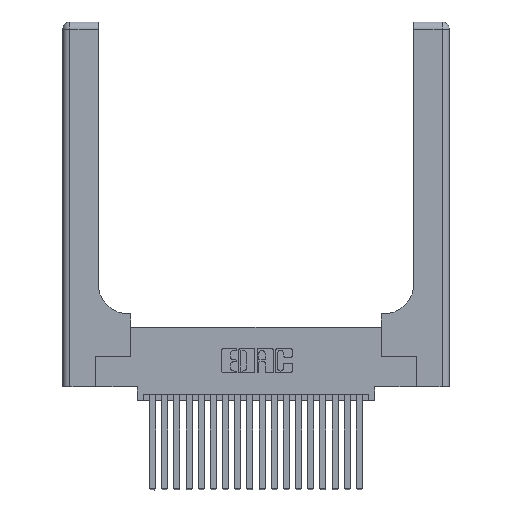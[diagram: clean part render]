
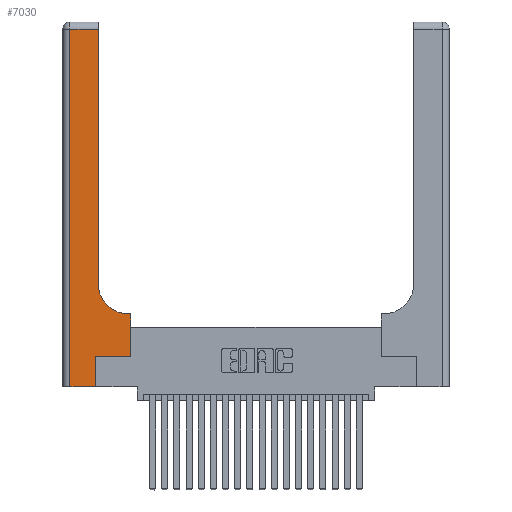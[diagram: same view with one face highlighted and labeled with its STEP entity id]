
A CAD part, top view. The second image highlights one B-rep face of the part: STEP entity #7030.
In plain terms, the highlighted planar face has unit normal (0, 0, 1).
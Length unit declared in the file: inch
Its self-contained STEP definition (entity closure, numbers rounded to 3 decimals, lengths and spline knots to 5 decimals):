
#413 = EDGE_CURVE ( 'NONE', #3244, #18240, #7618, .T. ) ;
#979 = DIRECTION ( 'NONE',  ( 0., 0., -1. ) ) ;
#2096 = CARTESIAN_POINT ( 'NONE',  ( 0.2915, 0.6, 0.37 ) ) ;
#2308 = DIRECTION ( 'NONE',  ( 0., 0., -1. ) ) ;
#2321 = DIRECTION ( 'NONE',  ( 0., 1., 0. ) ) ;
#3053 = EDGE_CURVE ( 'NONE', #18240, #21819, #3371, .T. ) ;
#3215 = EDGE_CURVE ( 'NONE', #21819, #20102, #10783, .T. ) ;
#3244 = VERTEX_POINT ( 'NONE', #16145 ) ;
#3371 = LINE ( 'NONE', #14045, #15663 ) ;
#3552 = VERTEX_POINT ( 'NONE', #8536 ) ;
#3729 = CARTESIAN_POINT ( 'NONE',  ( 0.269, 0., 0.37 ) ) ;
#3808 = DIRECTION ( 'NONE',  ( 0., 1., 0. ) ) ;
#4030 = LINE ( 'NONE', #7240, #22029 ) ;
#4136 = DIRECTION ( 'NONE',  ( -1., 0., 0. ) ) ;
#4292 = CARTESIAN_POINT ( 'NONE',  ( 0.2915, 0.85, 0.37 ) ) ;
#4666 = VERTEX_POINT ( 'NONE', #6856 ) ;
#5130 = CIRCLE ( 'NONE', #10018, 0.25 ) ;
#5564 = LINE ( 'NONE', #19434, #20297 ) ;
#5689 = CARTESIAN_POINT ( 'NONE',  ( 0., 0., 0.37 ) ) ;
#5730 = CARTESIAN_POINT ( 'NONE',  ( 0., 3., 0.37 ) ) ;
#6856 = CARTESIAN_POINT ( 'NONE',  ( 0.5415, 0.6, 0.37 ) ) ;
#7030 = ADVANCED_FACE ( 'NONE', ( #18524 ), #19592, .F. ) ;
#7106 = DIRECTION ( 'NONE',  ( 0., -1., 0. ) ) ;
#7137 = ORIENTED_EDGE ( 'NONE', *, *, #3215, .T. ) ;
#7147 = EDGE_CURVE ( 'NONE', #14586, #3244, #19969, .T. ) ;
#7240 = CARTESIAN_POINT ( 'NONE',  ( 0.269, 0., 0.37 ) ) ;
#7618 = LINE ( 'NONE', #19532, #13904 ) ;
#7993 = VECTOR ( 'NONE', #19079, 39.37008 ) ;
#8536 = CARTESIAN_POINT ( 'NONE',  ( 0.269, 0.25, 0.37 ) ) ;
#8881 = ORIENTED_EDGE ( 'NONE', *, *, #9396, .T. ) ;
#9396 = EDGE_CURVE ( 'NONE', #20102, #3552, #4030, .T. ) ;
#10013 = CARTESIAN_POINT ( 'NONE',  ( 0.5415, 0.85, 0.37 ) ) ;
#10018 = AXIS2_PLACEMENT_3D ( 'NONE', #10013, #979, #18558 ) ;
#10308 = ORIENTED_EDGE ( 'NONE', *, *, #413, .T. ) ;
#10516 = VECTOR ( 'NONE', #17870, 39.37008 ) ;
#10616 = EDGE_CURVE ( 'NONE', #3552, #20323, #14424, .T. ) ;
#10783 = LINE ( 'NONE', #5689, #10516 ) ;
#11332 = CARTESIAN_POINT ( 'NONE',  ( 0.5585, 0.25, 0.37 ) ) ;
#11626 = DIRECTION ( 'NONE',  ( 1., 0., 0. ) ) ;
#12137 = CARTESIAN_POINT ( 'NONE',  ( 0.2915, 3., 0.37 ) ) ;
#13302 = CARTESIAN_POINT ( 'NONE',  ( 0.269, 0.25, 0.37 ) ) ;
#13904 = VECTOR ( 'NONE', #4136, 39.37008 ) ;
#13952 = CARTESIAN_POINT ( 'NONE',  ( 0.5585, 0.6, 0.37 ) ) ;
#14045 = CARTESIAN_POINT ( 'NONE',  ( 0.06, 3., 0.37 ) ) ;
#14312 = DIRECTION ( 'NONE',  ( -1., 0., 0. ) ) ;
#14424 = LINE ( 'NONE', #13302, #22014 ) ;
#14464 = CARTESIAN_POINT ( 'NONE',  ( 0.06, 0., 0.37 ) ) ;
#14515 = DIRECTION ( 'NONE',  ( -1., 0., 0. ) ) ;
#14586 = VERTEX_POINT ( 'NONE', #4292 ) ;
#14975 = EDGE_CURVE ( 'NONE', #20323, #19308, #5564, .T. ) ;
#15663 = VECTOR ( 'NONE', #7106, 39.37008 ) ;
#16113 = AXIS2_PLACEMENT_3D ( 'NONE', #5730, #2308, #14515 ) ;
#16135 = VECTOR ( 'NONE', #14312, 39.37008 ) ;
#16145 = CARTESIAN_POINT ( 'NONE',  ( 0.2915, 2.94, 0.37 ) ) ;
#17010 = ORIENTED_EDGE ( 'NONE', *, *, #21442, .T. ) ;
#17870 = DIRECTION ( 'NONE',  ( 1., 0., 0. ) ) ;
#17898 = ORIENTED_EDGE ( 'NONE', *, *, #10616, .T. ) ;
#18240 = VERTEX_POINT ( 'NONE', #19254 ) ;
#18406 = ORIENTED_EDGE ( 'NONE', *, *, #3053, .T. ) ;
#18524 = FACE_OUTER_BOUND ( 'NONE', #22319, .T. ) ;
#18531 = EDGE_CURVE ( 'NONE', #4666, #14586, #5130, .T. ) ;
#18558 = DIRECTION ( 'NONE',  ( 1., 0., 0. ) ) ;
#19050 = ORIENTED_EDGE ( 'NONE', *, *, #18531, .T. ) ;
#19079 = DIRECTION ( 'NONE',  ( 0., 1., 0. ) ) ;
#19254 = CARTESIAN_POINT ( 'NONE',  ( 0.06, 2.94, 0.37 ) ) ;
#19308 = VERTEX_POINT ( 'NONE', #13952 ) ;
#19434 = CARTESIAN_POINT ( 'NONE',  ( 0.5585, 0.25, 0.37 ) ) ;
#19532 = CARTESIAN_POINT ( 'NONE',  ( 0., 2.94, 0.37 ) ) ;
#19592 = PLANE ( 'NONE',  #16113 ) ;
#19969 = LINE ( 'NONE', #12137, #7993 ) ;
#20102 = VERTEX_POINT ( 'NONE', #3729 ) ;
#20297 = VECTOR ( 'NONE', #3808, 39.37008 ) ;
#20323 = VERTEX_POINT ( 'NONE', #11332 ) ;
#20532 = ORIENTED_EDGE ( 'NONE', *, *, #14975, .T. ) ;
#20743 = LINE ( 'NONE', #2096, #16135 ) ;
#20868 = ORIENTED_EDGE ( 'NONE', *, *, #7147, .T. ) ;
#21442 = EDGE_CURVE ( 'NONE', #19308, #4666, #20743, .T. ) ;
#21819 = VERTEX_POINT ( 'NONE', #14464 ) ;
#22014 = VECTOR ( 'NONE', #11626, 39.37008 ) ;
#22029 = VECTOR ( 'NONE', #2321, 39.37008 ) ;
#22319 = EDGE_LOOP ( 'NONE', ( #20868, #10308, #18406, #7137, #8881, #17898, #20532, #17010, #19050 ) ) ;
